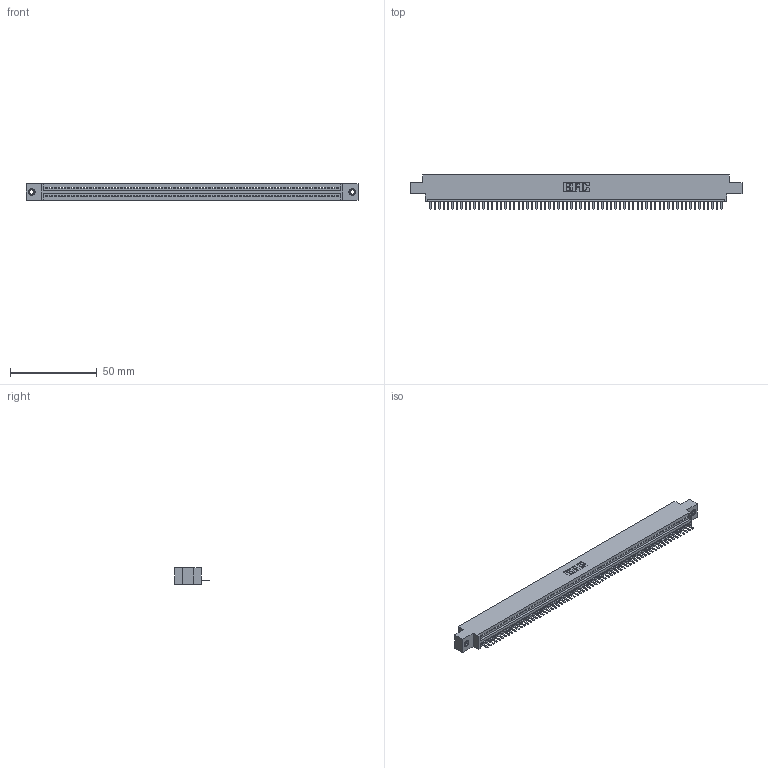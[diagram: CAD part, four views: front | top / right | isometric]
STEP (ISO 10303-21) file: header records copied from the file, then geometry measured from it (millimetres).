
FILE_DESCRIPTION (( 'STEP AP203' ), '1' );
FILE_NAME ('345-067-520-607.STEP', '2019-10-12T00:10:15', ( '' ), ( '' ), 'SwSTEP 2.0', 'SolidWorks 2016', '' );
FILE_SCHEMA (( 'CONFIG_CONTROL_DESIGN' ));
Length unit declared in the file: inch
Products named in the file (4): 345 Part_0.170 Offset - 0.156 Dia-TI; 345-250-001_345-250-005-103; 345-292-001_345-293-120; 345-067-520-607
Assembly tree (70 placements, depth 2):
  345-067-520-607
    345 Part_0.170 Offset - 0.156 Dia-TI
    345-292-001_345-293-120  x67
    345-250-001_345-250-005-103  x2
Bounding box: 191.39 x 19.68 x 9.4 mm (x, y, z)
Volume: 18063.5 mm3; surface area: 23873.1 mm2
Topology: 70 solids, 70 shells, 4344 faces, 12817 edges, 8358 vertices
Faces by surface type: plane 2930, cylinder 1398, cone 12, torus 4
Entity records: 48492 total; most frequent: CARTESIAN_POINT 8392, ORIENTED_EDGE 8374, DIRECTION 7307, EDGE_CURVE 4187, VECTOR 3763, LINE 3763, VERTEX_POINT 2784, AXIS2_PLACEMENT_3D 1772
